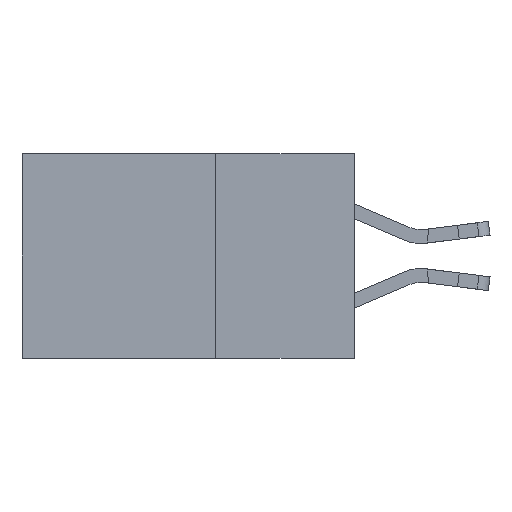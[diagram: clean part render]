
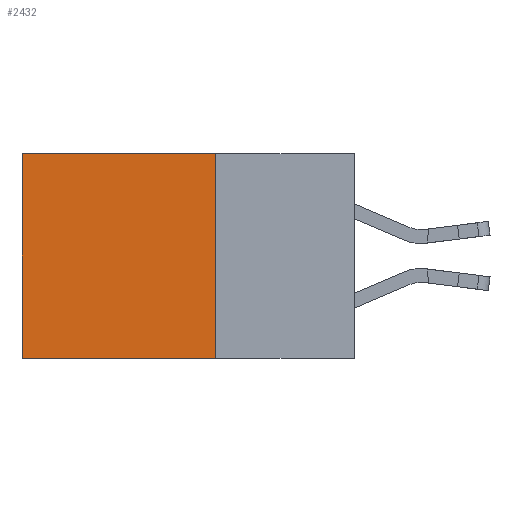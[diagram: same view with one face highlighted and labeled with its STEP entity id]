
A CAD part, left-side view. The second image highlights one B-rep face of the part: STEP entity #2432.
In plain terms, the highlighted planar face has unit normal (-1, 0, 0).
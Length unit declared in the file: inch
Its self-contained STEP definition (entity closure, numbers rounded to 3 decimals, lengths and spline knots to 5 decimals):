
#190 = EDGE_CURVE ( 'NONE', #9915, #6237, #11163, .T. ) ;
#763 = LINE ( 'NONE', #4416, #12150 ) ;
#864 = CARTESIAN_POINT ( 'NONE',  ( 0.298, 0.6, 0. ) ) ;
#1185 = DIRECTION ( 'NONE',  ( 0., 1., 0. ) ) ;
#1776 = DIRECTION ( 'NONE',  ( 0., 0., -1. ) ) ;
#2020 = CARTESIAN_POINT ( 'NONE',  ( 0.298, 0.25, 0. ) ) ;
#2280 = DIRECTION ( 'NONE',  ( 0., 0., -1. ) ) ;
#2432 = ADVANCED_FACE ( 'NONE', ( #7361 ), #11949, .F. ) ;
#3140 = EDGE_CURVE ( 'NONE', #6237, #6884, #763, .T. ) ;
#4277 = ORIENTED_EDGE ( 'NONE', *, *, #13529, .T. ) ;
#4416 = CARTESIAN_POINT ( 'NONE',  ( 0.298, 0.25, -0.37 ) ) ;
#4544 = EDGE_CURVE ( 'NONE', #9915, #7088, #14060, .T. ) ;
#4685 = VECTOR ( 'NONE', #6447, 39.37008 ) ;
#4690 = ORIENTED_EDGE ( 'NONE', *, *, #3140, .F. ) ;
#5088 = DIRECTION ( 'NONE',  ( 1., 0., 0. ) ) ;
#6237 = VERTEX_POINT ( 'NONE', #8076 ) ;
#6278 = CARTESIAN_POINT ( 'NONE',  ( 0.298, 0.25, 0. ) ) ;
#6447 = DIRECTION ( 'NONE',  ( 0., 1., 0. ) ) ;
#6488 = ORIENTED_EDGE ( 'NONE', *, *, #4544, .T. ) ;
#6884 = VERTEX_POINT ( 'NONE', #12384 ) ;
#7088 = VERTEX_POINT ( 'NONE', #864 ) ;
#7361 = FACE_OUTER_BOUND ( 'NONE', #11644, .T. ) ;
#8076 = CARTESIAN_POINT ( 'NONE',  ( 0.298, 0.25, -0.37 ) ) ;
#9064 = CARTESIAN_POINT ( 'NONE',  ( 0.298, 0.6, 0. ) ) ;
#9357 = VECTOR ( 'NONE', #2280, 39.37008 ) ;
#9915 = VERTEX_POINT ( 'NONE', #14021 ) ;
#10738 = ORIENTED_EDGE ( 'NONE', *, *, #190, .F. ) ;
#11163 = LINE ( 'NONE', #14466, #13857 ) ;
#11644 = EDGE_LOOP ( 'NONE', ( #4277, #4690, #10738, #6488 ) ) ;
#11949 = PLANE ( 'NONE',  #14098 ) ;
#12150 = VECTOR ( 'NONE', #1185, 39.37008 ) ;
#12265 = DIRECTION ( 'NONE',  ( 0., 0., -1. ) ) ;
#12384 = CARTESIAN_POINT ( 'NONE',  ( 0.298, 0.6, -0.37 ) ) ;
#12759 = LINE ( 'NONE', #9064, #9357 ) ;
#13529 = EDGE_CURVE ( 'NONE', #7088, #6884, #12759, .T. ) ;
#13857 = VECTOR ( 'NONE', #12265, 39.37008 ) ;
#14021 = CARTESIAN_POINT ( 'NONE',  ( 0.298, 0.25, 0. ) ) ;
#14060 = LINE ( 'NONE', #2020, #4685 ) ;
#14098 = AXIS2_PLACEMENT_3D ( 'NONE', #6278, #5088, #1776 ) ;
#14466 = CARTESIAN_POINT ( 'NONE',  ( 0.298, 0.25, 0. ) ) ;
